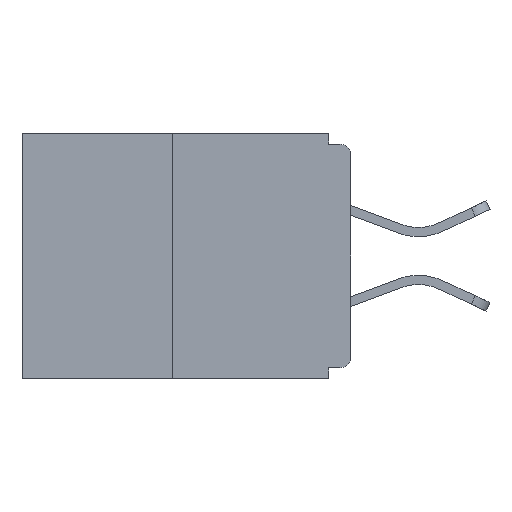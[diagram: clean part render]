
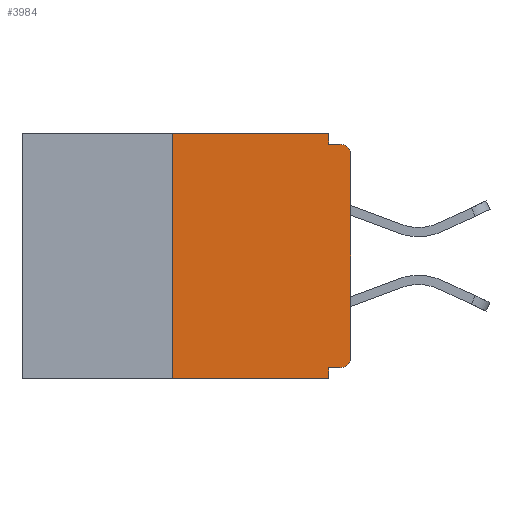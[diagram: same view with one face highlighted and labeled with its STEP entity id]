
A CAD part, left-side view. The second image highlights one B-rep face of the part: STEP entity #3984.
In plain terms, the highlighted planar face has unit normal (-1, 0, 0).
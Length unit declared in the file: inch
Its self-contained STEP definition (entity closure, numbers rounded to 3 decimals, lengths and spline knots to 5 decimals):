
#295 = ORIENTED_EDGE ( 'NONE', *, *, #19945, .F. ) ;
#381 = ORIENTED_EDGE ( 'NONE', *, *, #18908, .F. ) ;
#747 = EDGE_CURVE ( 'NONE', #18347, #21466, #15183, .T. ) ;
#782 = ORIENTED_EDGE ( 'NONE', *, *, #3769, .F. ) ;
#1110 = EDGE_LOOP ( 'NONE', ( #6075, #381, #15195, #10253, #782, #8880, #15750, #14596, #295, #4742 ) ) ;
#1389 = DIRECTION ( 'NONE',  ( 0., 0., -1. ) ) ;
#1668 = DIRECTION ( 'NONE',  ( 0., 0., -1. ) ) ;
#1683 = VERTEX_POINT ( 'NONE', #15379 ) ;
#2382 = DIRECTION ( 'NONE',  ( 1., 0., 0. ) ) ;
#2964 = CARTESIAN_POINT ( 'NONE',  ( 0., 0.015, -0.313 ) ) ;
#3126 = EDGE_CURVE ( 'NONE', #18590, #14293, #5723, .T. ) ;
#3149 = CARTESIAN_POINT ( 'NONE',  ( 0., 0., 0. ) ) ;
#3428 = CARTESIAN_POINT ( 'NONE',  ( 0., 0.031, -0.328 ) ) ;
#3707 = LINE ( 'NONE', #11793, #21262 ) ;
#3769 = EDGE_CURVE ( 'NONE', #18347, #21651, #5209, .T. ) ;
#3908 = LINE ( 'NONE', #9598, #16689 ) ;
#3984 = ADVANCED_FACE ( 'NONE', ( #7847 ), #5761, .F. ) ;
#4742 = ORIENTED_EDGE ( 'NONE', *, *, #9552, .F. ) ;
#4867 = DIRECTION ( 'NONE',  ( 0., -1., 0. ) ) ;
#5012 = CARTESIAN_POINT ( 'NONE',  ( 0., 0.031, -0.343 ) ) ;
#5209 = LINE ( 'NONE', #17965, #20356 ) ;
#5497 = CARTESIAN_POINT ( 'NONE',  ( 0., 0.25, -0.343 ) ) ;
#5723 = LINE ( 'NONE', #14360, #9162 ) ;
#5761 = PLANE ( 'NONE',  #7458 ) ;
#6075 = ORIENTED_EDGE ( 'NONE', *, *, #9075, .F. ) ;
#6222 = DIRECTION ( 'NONE',  ( 0., 1., 0. ) ) ;
#6391 = CARTESIAN_POINT ( 'NONE',  ( 0., 0.031, 0. ) ) ;
#7458 = AXIS2_PLACEMENT_3D ( 'NONE', #12590, #2382, #21136 ) ;
#7688 = DIRECTION ( 'NONE',  ( 0., 0., -1. ) ) ;
#7847 = FACE_OUTER_BOUND ( 'NONE', #1110, .T. ) ;
#7858 = EDGE_CURVE ( 'NONE', #21466, #9974, #9902, .T. ) ;
#8392 = VERTEX_POINT ( 'NONE', #18461 ) ;
#8799 = VERTEX_POINT ( 'NONE', #20652 ) ;
#8880 = ORIENTED_EDGE ( 'NONE', *, *, #747, .T. ) ;
#9075 = EDGE_CURVE ( 'NONE', #8392, #1683, #14113, .T. ) ;
#9162 = VECTOR ( 'NONE', #17621, 39.37008 ) ;
#9439 = DIRECTION ( 'NONE',  ( -1., 0., 0. ) ) ;
#9552 = EDGE_CURVE ( 'NONE', #1683, #20436, #11661, .T. ) ;
#9598 = CARTESIAN_POINT ( 'NONE',  ( 0., 0.031, -0.343 ) ) ;
#9791 = VECTOR ( 'NONE', #1668, 39.37008 ) ;
#9902 = LINE ( 'NONE', #3149, #11769 ) ;
#9974 = VERTEX_POINT ( 'NONE', #15319 ) ;
#10253 = ORIENTED_EDGE ( 'NONE', *, *, #14822, .F. ) ;
#10805 = CARTESIAN_POINT ( 'NONE',  ( 0., 0., -0.313 ) ) ;
#11661 = LINE ( 'NONE', #6391, #9791 ) ;
#11769 = VECTOR ( 'NONE', #13533, 39.37008 ) ;
#11793 = CARTESIAN_POINT ( 'NONE',  ( 0., 0.25, 0. ) ) ;
#12590 = CARTESIAN_POINT ( 'NONE',  ( 0., 0.46, 0. ) ) ;
#13517 = DIRECTION ( 'NONE',  ( 0., 0., 1. ) ) ;
#13533 = DIRECTION ( 'NONE',  ( 0., 0., 1. ) ) ;
#14055 = VECTOR ( 'NONE', #4867, 39.37008 ) ;
#14113 = LINE ( 'NONE', #17214, #17293 ) ;
#14293 = VERTEX_POINT ( 'NONE', #5012 ) ;
#14360 = CARTESIAN_POINT ( 'NONE',  ( 0., 0.46, -0.343 ) ) ;
#14596 = ORIENTED_EDGE ( 'NONE', *, *, #21004, .T. ) ;
#14822 = EDGE_CURVE ( 'NONE', #21651, #14293, #3908, .T. ) ;
#14906 = DIRECTION ( 'NONE',  ( -1., 0., 0. ) ) ;
#15183 = CIRCLE ( 'NONE', #16394, 0.015 ) ;
#15195 = ORIENTED_EDGE ( 'NONE', *, *, #3126, .T. ) ;
#15319 = CARTESIAN_POINT ( 'NONE',  ( 0., 0., -0.03 ) ) ;
#15379 = CARTESIAN_POINT ( 'NONE',  ( 0., 0.031, 0. ) ) ;
#15750 = ORIENTED_EDGE ( 'NONE', *, *, #7858, .T. ) ;
#16394 = AXIS2_PLACEMENT_3D ( 'NONE', #2964, #14906, #1389 ) ;
#16610 = AXIS2_PLACEMENT_3D ( 'NONE', #19782, #9439, #21352 ) ;
#16689 = VECTOR ( 'NONE', #7688, 39.37008 ) ;
#16940 = CIRCLE ( 'NONE', #16610, 0.015 ) ;
#17214 = CARTESIAN_POINT ( 'NONE',  ( 0., 0.46, 0. ) ) ;
#17293 = VECTOR ( 'NONE', #17429, 39.37008 ) ;
#17429 = DIRECTION ( 'NONE',  ( 0., -1., 0. ) ) ;
#17621 = DIRECTION ( 'NONE',  ( 0., -1., 0. ) ) ;
#17918 = CARTESIAN_POINT ( 'NONE',  ( 0., 0.031, -0.015 ) ) ;
#17965 = CARTESIAN_POINT ( 'NONE',  ( 0., 0., -0.328 ) ) ;
#18347 = VERTEX_POINT ( 'NONE', #21714 ) ;
#18461 = CARTESIAN_POINT ( 'NONE',  ( 0., 0.25, 0. ) ) ;
#18590 = VERTEX_POINT ( 'NONE', #5497 ) ;
#18830 = LINE ( 'NONE', #22094, #14055 ) ;
#18908 = EDGE_CURVE ( 'NONE', #18590, #8392, #3707, .T. ) ;
#19782 = CARTESIAN_POINT ( 'NONE',  ( 0., 0.015, -0.03 ) ) ;
#19945 = EDGE_CURVE ( 'NONE', #20436, #8799, #18830, .T. ) ;
#20356 = VECTOR ( 'NONE', #6222, 39.37008 ) ;
#20436 = VERTEX_POINT ( 'NONE', #17918 ) ;
#20652 = CARTESIAN_POINT ( 'NONE',  ( 0., 0.015, -0.015 ) ) ;
#21004 = EDGE_CURVE ( 'NONE', #9974, #8799, #16940, .T. ) ;
#21136 = DIRECTION ( 'NONE',  ( 0., 0., -1. ) ) ;
#21262 = VECTOR ( 'NONE', #13517, 39.37008 ) ;
#21352 = DIRECTION ( 'NONE',  ( 0., 0., -1. ) ) ;
#21466 = VERTEX_POINT ( 'NONE', #10805 ) ;
#21651 = VERTEX_POINT ( 'NONE', #3428 ) ;
#21714 = CARTESIAN_POINT ( 'NONE',  ( 0., 0.015, -0.328 ) ) ;
#22094 = CARTESIAN_POINT ( 'NONE',  ( 0., 0., -0.015 ) ) ;
